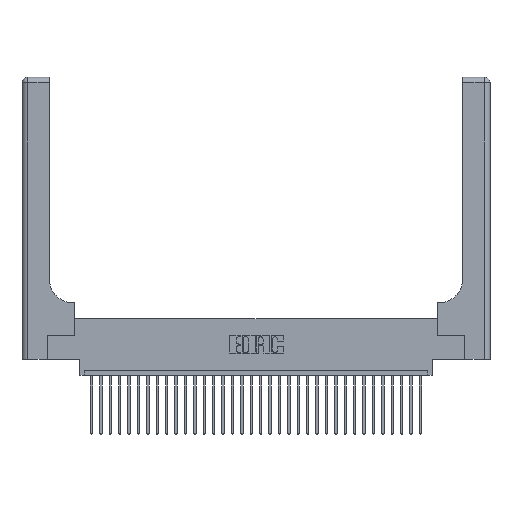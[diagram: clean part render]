
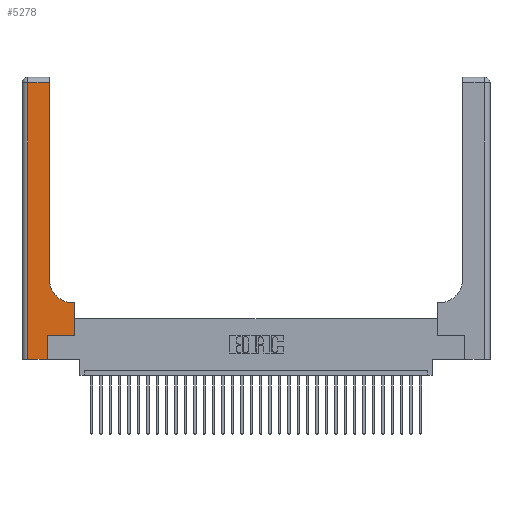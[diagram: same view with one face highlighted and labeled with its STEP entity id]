
A CAD part, top view. The second image highlights one B-rep face of the part: STEP entity #5278.
In plain terms, the highlighted planar face has unit normal (0, 0, 1).
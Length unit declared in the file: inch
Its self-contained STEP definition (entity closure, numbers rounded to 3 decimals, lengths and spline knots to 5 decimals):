
#239 = ORIENTED_EDGE ( 'NONE', *, *, #12093, .T. ) ;
#588 = CARTESIAN_POINT ( 'NONE',  ( 0.2915, 0.85, 0.37 ) ) ;
#958 = CARTESIAN_POINT ( 'NONE',  ( 0.06, 3., 0.37 ) ) ;
#1286 = CARTESIAN_POINT ( 'NONE',  ( 0.2915, 3., 0.37 ) ) ;
#1509 = VECTOR ( 'NONE', #17273, 39.37008 ) ;
#1739 = VECTOR ( 'NONE', #2187, 39.37008 ) ;
#1829 = ORIENTED_EDGE ( 'NONE', *, *, #9566, .T. ) ;
#2187 = DIRECTION ( 'NONE',  ( -1., 0., 0. ) ) ;
#2455 = ORIENTED_EDGE ( 'NONE', *, *, #3393, .T. ) ;
#2823 = ORIENTED_EDGE ( 'NONE', *, *, #26153, .T. ) ;
#3393 = EDGE_CURVE ( 'NONE', #19233, #5621, #14493, .T. ) ;
#3790 = CARTESIAN_POINT ( 'NONE',  ( 0.5415, 0.85, 0.37 ) ) ;
#3932 = EDGE_CURVE ( 'NONE', #20399, #9494, #27556, .T. ) ;
#4613 = ORIENTED_EDGE ( 'NONE', *, *, #29106, .T. ) ;
#4671 = CARTESIAN_POINT ( 'NONE',  ( 0.269, 0.25, 0.37 ) ) ;
#5278 = ADVANCED_FACE ( 'NONE', ( #21004 ), #27159, .F. ) ;
#5537 = CIRCLE ( 'NONE', #7770, 0.25 ) ;
#5621 = VERTEX_POINT ( 'NONE', #21607 ) ;
#6165 = AXIS2_PLACEMENT_3D ( 'NONE', #22374, #12183, #24477 ) ;
#6967 = DIRECTION ( 'NONE',  ( 0., 1., 0. ) ) ;
#7192 = LINE ( 'NONE', #17619, #1509 ) ;
#7363 = DIRECTION ( 'NONE',  ( 0., 1., 0. ) ) ;
#7770 = AXIS2_PLACEMENT_3D ( 'NONE', #3790, #24563, #11812 ) ;
#8138 = ORIENTED_EDGE ( 'NONE', *, *, #9416, .T. ) ;
#8773 = LINE ( 'NONE', #4671, #16776 ) ;
#9416 = EDGE_CURVE ( 'NONE', #31137, #14372, #5537, .T. ) ;
#9494 = VERTEX_POINT ( 'NONE', #29921 ) ;
#9566 = EDGE_CURVE ( 'NONE', #9494, #19233, #7192, .T. ) ;
#9907 = CARTESIAN_POINT ( 'NONE',  ( 0., 2.94, 0.37 ) ) ;
#10588 = VECTOR ( 'NONE', #7363, 39.37008 ) ;
#11427 = VERTEX_POINT ( 'NONE', #18221 ) ;
#11812 = DIRECTION ( 'NONE',  ( 1., 0., 0. ) ) ;
#12088 = EDGE_CURVE ( 'NONE', #14372, #14736, #22251, .T. ) ;
#12093 = EDGE_CURVE ( 'NONE', #21901, #31137, #25827, .T. ) ;
#12183 = DIRECTION ( 'NONE',  ( 0., 0., -1. ) ) ;
#14372 = VERTEX_POINT ( 'NONE', #588 ) ;
#14493 = LINE ( 'NONE', #22752, #26482 ) ;
#14736 = VERTEX_POINT ( 'NONE', #16268 ) ;
#15002 = CARTESIAN_POINT ( 'NONE',  ( 0.2915, 0.6, 0.37 ) ) ;
#15206 = VECTOR ( 'NONE', #32960, 39.37008 ) ;
#15423 = VECTOR ( 'NONE', #6967, 39.37008 ) ;
#16268 = CARTESIAN_POINT ( 'NONE',  ( 0.2915, 2.94, 0.37 ) ) ;
#16776 = VECTOR ( 'NONE', #30146, 39.37008 ) ;
#17039 = DIRECTION ( 'NONE',  ( 0., -1., 0. ) ) ;
#17273 = DIRECTION ( 'NONE',  ( 1., 0., 0. ) ) ;
#17619 = CARTESIAN_POINT ( 'NONE',  ( 0., 0., 0.37 ) ) ;
#17877 = CARTESIAN_POINT ( 'NONE',  ( 0.5585, 0.25, 0.37 ) ) ;
#18221 = CARTESIAN_POINT ( 'NONE',  ( 0.5585, 0.25, 0.37 ) ) ;
#18541 = ORIENTED_EDGE ( 'NONE', *, *, #12088, .T. ) ;
#19060 = CARTESIAN_POINT ( 'NONE',  ( 0.06, 2.94, 0.37 ) ) ;
#19233 = VERTEX_POINT ( 'NONE', #21546 ) ;
#19894 = CARTESIAN_POINT ( 'NONE',  ( 0.5585, 0.6, 0.37 ) ) ;
#20399 = VERTEX_POINT ( 'NONE', #19060 ) ;
#21004 = FACE_OUTER_BOUND ( 'NONE', #27755, .T. ) ;
#21276 = CARTESIAN_POINT ( 'NONE',  ( 0.5415, 0.6, 0.37 ) ) ;
#21516 = VECTOR ( 'NONE', #17039, 39.37008 ) ;
#21546 = CARTESIAN_POINT ( 'NONE',  ( 0.269, 0., 0.37 ) ) ;
#21607 = CARTESIAN_POINT ( 'NONE',  ( 0.269, 0.25, 0.37 ) ) ;
#21901 = VERTEX_POINT ( 'NONE', #19894 ) ;
#22251 = LINE ( 'NONE', #1286, #15423 ) ;
#22374 = CARTESIAN_POINT ( 'NONE',  ( 0., 3., 0.37 ) ) ;
#22752 = CARTESIAN_POINT ( 'NONE',  ( 0.269, 0., 0.37 ) ) ;
#24477 = DIRECTION ( 'NONE',  ( -1., 0., 0. ) ) ;
#24563 = DIRECTION ( 'NONE',  ( 0., 0., -1. ) ) ;
#25827 = LINE ( 'NONE', #15002, #1739 ) ;
#26153 = EDGE_CURVE ( 'NONE', #5621, #11427, #8773, .T. ) ;
#26482 = VECTOR ( 'NONE', #27450, 39.37008 ) ;
#27159 = PLANE ( 'NONE',  #6165 ) ;
#27450 = DIRECTION ( 'NONE',  ( 0., 1., 0. ) ) ;
#27556 = LINE ( 'NONE', #958, #21516 ) ;
#27755 = EDGE_LOOP ( 'NONE', ( #18541, #29577, #31749, #1829, #2455, #2823, #4613, #239, #8138 ) ) ;
#29106 = EDGE_CURVE ( 'NONE', #11427, #21901, #31000, .T. ) ;
#29186 = LINE ( 'NONE', #9907, #15206 ) ;
#29577 = ORIENTED_EDGE ( 'NONE', *, *, #29782, .T. ) ;
#29782 = EDGE_CURVE ( 'NONE', #14736, #20399, #29186, .T. ) ;
#29921 = CARTESIAN_POINT ( 'NONE',  ( 0.06, 0., 0.37 ) ) ;
#30146 = DIRECTION ( 'NONE',  ( 1., 0., 0. ) ) ;
#31000 = LINE ( 'NONE', #17877, #10588 ) ;
#31137 = VERTEX_POINT ( 'NONE', #21276 ) ;
#31749 = ORIENTED_EDGE ( 'NONE', *, *, #3932, .T. ) ;
#32960 = DIRECTION ( 'NONE',  ( -1., 0., 0. ) ) ;
